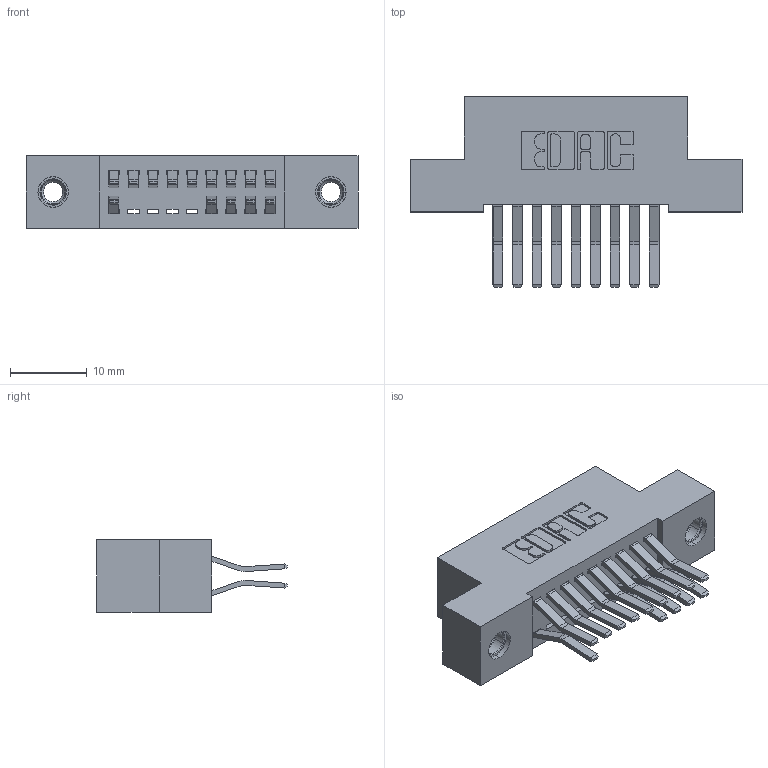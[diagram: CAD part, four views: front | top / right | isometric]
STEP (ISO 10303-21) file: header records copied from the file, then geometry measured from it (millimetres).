
FILE_DESCRIPTION (( 'STEP AP203' ), '1' );
FILE_NAME ('392-018-560-207.STEP', '2018-08-15T05:03:35', ( '' ), ( '' ), 'SwSTEP 2.0', 'SolidWorks 2016', '' );
FILE_SCHEMA (( 'CONFIG_CONTROL_DESIGN' ));
Length unit declared in the file: inch
Products named in the file (4): 345-250-001_345-250-005-103; 392-018-560-207; 342 Part_TI; 345-292-001_560 Tail
Assembly tree (17 placements, depth 2):
  392-018-560-207
    342 Part_TI
    345-292-001_560 Tail  x14
    345-250-001_345-250-005-103  x2
Bounding box: 43.18 x 24.78 x 9.4 mm (x, y, z)
Volume: 3766.8 mm3; surface area: 5365.4 mm2
Topology: 17 solids, 17 shells, 950 faces, 2773 edges, 1822 vertices
Faces by surface type: plane 626, cylinder 308, cone 12, torus 4
Entity records: 11072 total; most frequent: CARTESIAN_POINT 1873, ORIENTED_EDGE 1806, DIRECTION 1689, EDGE_CURVE 903, LINE 751, VECTOR 751, VERTEX_POINT 596, AXIS2_PLACEMENT_3D 469
